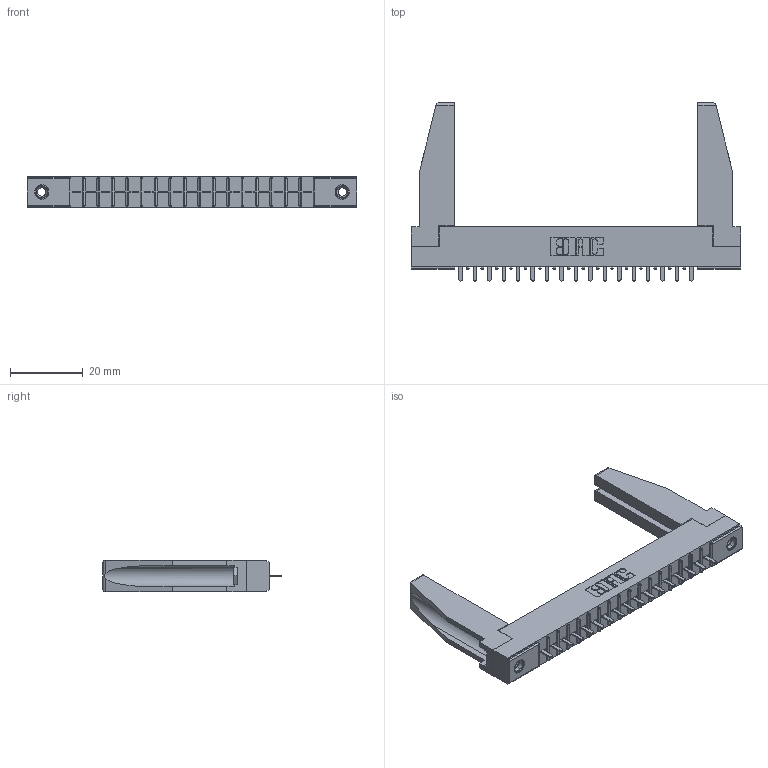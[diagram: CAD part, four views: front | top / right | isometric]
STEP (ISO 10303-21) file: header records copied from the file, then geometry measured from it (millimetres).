
FILE_DESCRIPTION (( 'STEP AP203' ), '1' );
FILE_NAME ('316-017-521-178.STEP', '2018-07-31T01:12:10', ( '' ), ( '' ), 'SwSTEP 2.0', 'SolidWorks 2016', '' );
FILE_SCHEMA (( 'CONFIG_CONTROL_DESIGN' ));
Length unit declared in the file: inch
Products named in the file (5): 306 Part_.156 Dia; 306-290-001_121; 345-250-001_345-250-001-102; 307-220-078; 316-017-521-178
Assembly tree (22 placements, depth 2):
  316-017-521-178
    306 Part_.156 Dia
    306-290-001_121  x17
    345-250-001_345-250-001-102  x2
    307-220-078  x2
Bounding box: 90.37 x 48.92 x 8.71 mm (x, y, z)
Volume: 10134.2 mm3; surface area: 12623.3 mm2
Topology: 22 solids, 22 shells, 1436 faces, 3995 edges, 2562 vertices
Faces by surface type: plane 951, cylinder 401, sphere 68, cone 12, torus 4
Entity records: 21487 total; most frequent: CARTESIAN_POINT 3604, ORIENTED_EDGE 3528, DIRECTION 3508, EDGE_CURVE 1764, LINE 1368, VECTOR 1368, VERTEX_POINT 1124, AXIS2_PLACEMENT_3D 1070
